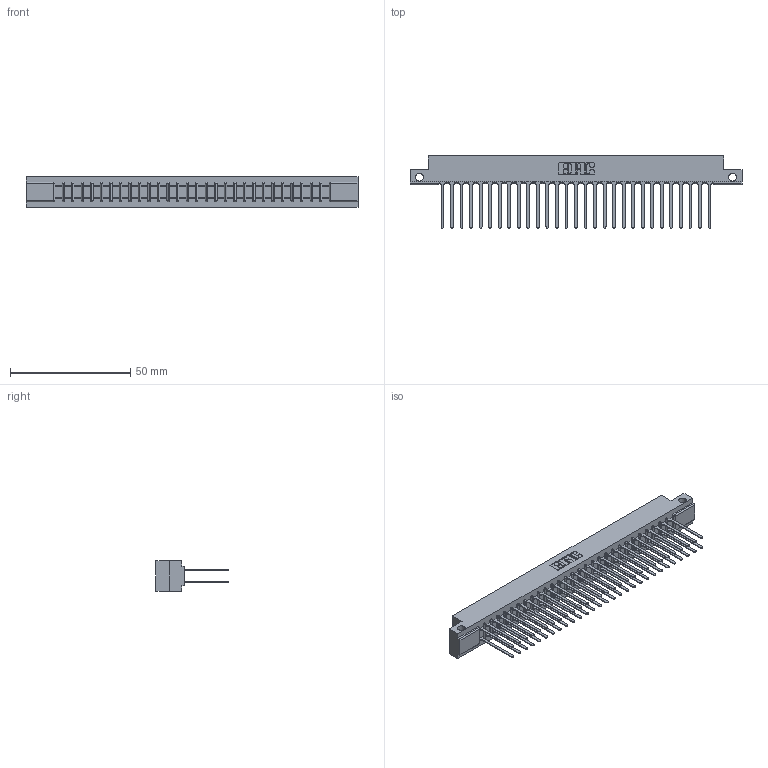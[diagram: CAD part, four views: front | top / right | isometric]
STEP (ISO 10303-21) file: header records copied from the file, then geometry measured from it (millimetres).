
FILE_DESCRIPTION (( 'STEP AP203' ), '1' );
FILE_NAME ('307-058-440-212.STEP', '2020-09-30T12:21:43', ( '' ), ( '' ), 'SwSTEP 2.0', 'SolidWorks 2020', '' );
FILE_SCHEMA (( 'CONFIG_CONTROL_DESIGN' ));
Length unit declared in the file: inch
Products named in the file (3): 307-290-001_540; 307-058-440-212; 307 Part_.128 Dia Side Mounting Holes
Assembly tree (59 placements, depth 2):
  307-058-440-212
    307 Part_.128 Dia Side Mounting Holes
    307-290-001_540  x58
Bounding box: 137.92 x 30 x 12.7 mm (x, y, z)
Volume: 14756 mm3; surface area: 19712.5 mm2
Topology: 59 solids, 59 shells, 2816 faces, 7863 edges, 5082 vertices
Faces by surface type: plane 1868, cylinder 888, sphere 60
Entity records: 27362 total; most frequent: CARTESIAN_POINT 4477, ORIENTED_EDGE 4434, DIRECTION 4391, EDGE_CURVE 2217, VECTOR 1695, LINE 1695, VERTEX_POINT 1434, AXIS2_PLACEMENT_3D 1348
